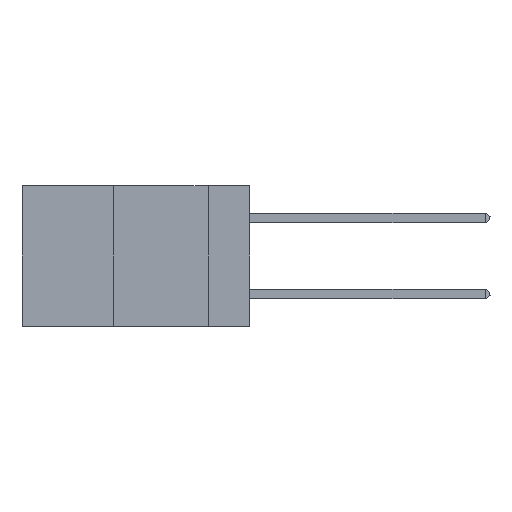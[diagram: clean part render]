
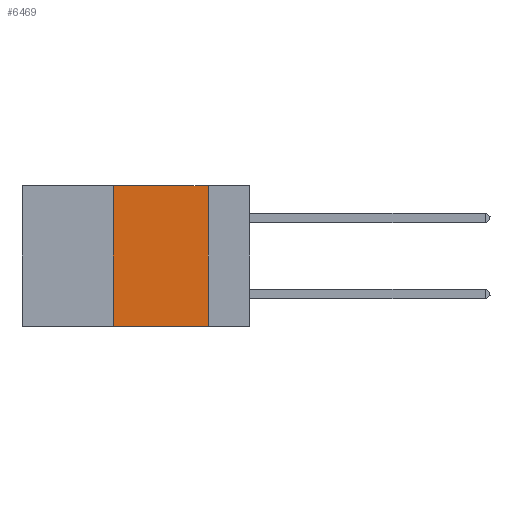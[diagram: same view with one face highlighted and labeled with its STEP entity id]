
A CAD part, left-side view. The second image highlights one B-rep face of the part: STEP entity #6469.
In plain terms, the highlighted planar face has unit normal (-1, 0, 0).
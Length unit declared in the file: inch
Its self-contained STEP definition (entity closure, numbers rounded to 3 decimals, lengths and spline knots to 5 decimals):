
#39 = CARTESIAN_POINT ( 'NONE',  ( 0., 0.11, 0. ) ) ;
#143 = VECTOR ( 'NONE', #20985, 39.37008 ) ;
#1672 = LINE ( 'NONE', #29626, #18599 ) ;
#2183 = LINE ( 'NONE', #3915, #2894 ) ;
#2550 = CARTESIAN_POINT ( 'NONE',  ( 0., 0.6, 0. ) ) ;
#2815 = FACE_OUTER_BOUND ( 'NONE', #14494, .T. ) ;
#2894 = VECTOR ( 'NONE', #15295, 39.37008 ) ;
#3532 = EDGE_CURVE ( 'NONE', #13695, #3718, #8729, .T. ) ;
#3718 = VERTEX_POINT ( 'NONE', #29678 ) ;
#3915 = CARTESIAN_POINT ( 'NONE',  ( 0., 0.6, -0.37 ) ) ;
#4077 = VECTOR ( 'NONE', #9307, 39.37008 ) ;
#5173 = EDGE_CURVE ( 'NONE', #27233, #3718, #2183, .T. ) ;
#6082 = VERTEX_POINT ( 'NONE', #25652 ) ;
#6236 = LINE ( 'NONE', #2550, #143 ) ;
#6469 = ADVANCED_FACE ( 'NONE', ( #2815 ), #11229, .F. ) ;
#6982 = CARTESIAN_POINT ( 'NONE',  ( 0., 0.11, 0. ) ) ;
#7543 = CARTESIAN_POINT ( 'NONE',  ( 0., 0.36, -0.37 ) ) ;
#8124 = AXIS2_PLACEMENT_3D ( 'NONE', #22870, #21033, #23365 ) ;
#8729 = LINE ( 'NONE', #6982, #4077 ) ;
#9307 = DIRECTION ( 'NONE',  ( 0., 0., -1. ) ) ;
#11229 = PLANE ( 'NONE',  #8124 ) ;
#13695 = VERTEX_POINT ( 'NONE', #39 ) ;
#14494 = EDGE_LOOP ( 'NONE', ( #22321, #22008, #26996, #28076 ) ) ;
#15295 = DIRECTION ( 'NONE',  ( 0., -1., 0. ) ) ;
#18599 = VECTOR ( 'NONE', #22777, 39.37008 ) ;
#20985 = DIRECTION ( 'NONE',  ( 0., -1., 0. ) ) ;
#21033 = DIRECTION ( 'NONE',  ( 1., 0., 0. ) ) ;
#22008 = ORIENTED_EDGE ( 'NONE', *, *, #26027, .F. ) ;
#22321 = ORIENTED_EDGE ( 'NONE', *, *, #3532, .F. ) ;
#22777 = DIRECTION ( 'NONE',  ( 0., 0., 1. ) ) ;
#22870 = CARTESIAN_POINT ( 'NONE',  ( 0., 0.6, 0. ) ) ;
#23365 = DIRECTION ( 'NONE',  ( 0., 0., -1. ) ) ;
#24685 = EDGE_CURVE ( 'NONE', #27233, #6082, #1672, .T. ) ;
#25652 = CARTESIAN_POINT ( 'NONE',  ( 0., 0.36, 0. ) ) ;
#26027 = EDGE_CURVE ( 'NONE', #6082, #13695, #6236, .T. ) ;
#26996 = ORIENTED_EDGE ( 'NONE', *, *, #24685, .F. ) ;
#27233 = VERTEX_POINT ( 'NONE', #7543 ) ;
#28076 = ORIENTED_EDGE ( 'NONE', *, *, #5173, .T. ) ;
#29626 = CARTESIAN_POINT ( 'NONE',  ( 0., 0.36, 0. ) ) ;
#29678 = CARTESIAN_POINT ( 'NONE',  ( 0., 0.11, -0.37 ) ) ;
